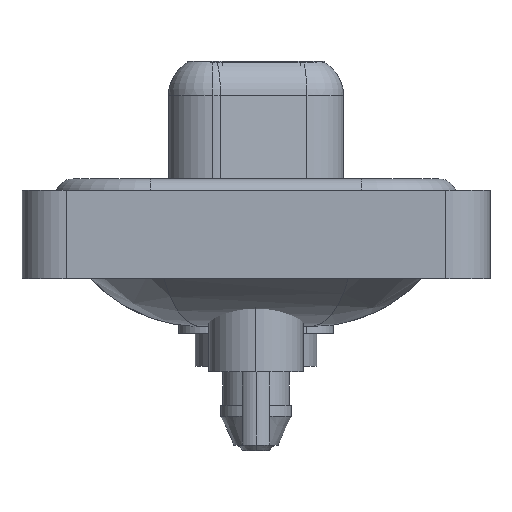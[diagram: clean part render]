
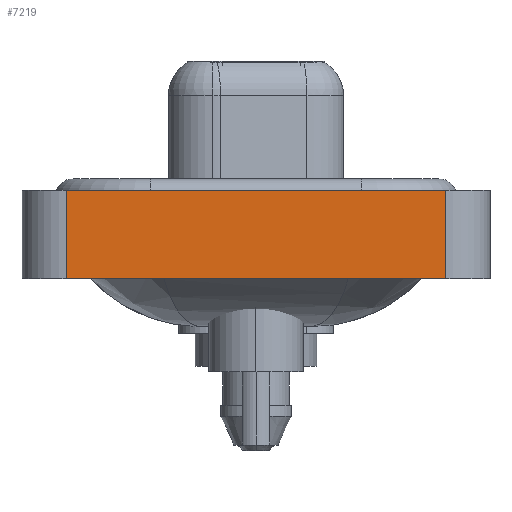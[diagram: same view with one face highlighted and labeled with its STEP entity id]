
A CAD part, left-side view. The second image highlights one B-rep face of the part: STEP entity #7219.
In plain terms, the highlighted planar face has unit normal (-1, 0, 0).
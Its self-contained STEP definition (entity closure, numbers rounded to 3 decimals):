
#433 = CARTESIAN_POINT ( 'NONE',  ( -7.25, 8.55, -3.6 ) ) ;
#957 = VERTEX_POINT ( 'NONE', #4955 ) ;
#996 = ORIENTED_EDGE ( 'NONE', *, *, #7742, .T. ) ;
#1111 = VERTEX_POINT ( 'NONE', #6572 ) ;
#1284 = FACE_OUTER_BOUND ( 'NONE', #15716, .T. ) ;
#1933 = VECTOR ( 'NONE', #14271, 1000. ) ;
#2251 = VERTEX_POINT ( 'NONE', #12895 ) ;
#2967 = CARTESIAN_POINT ( 'NONE',  ( -7.25, -8.55, -3.6 ) ) ;
#3525 = CARTESIAN_POINT ( 'NONE',  ( -7.25, -8.55, -3.6 ) ) ;
#4658 = CARTESIAN_POINT ( 'NONE',  ( -7.25, -8.55, 0.4 ) ) ;
#4955 = CARTESIAN_POINT ( 'NONE',  ( -7.25, -8.55, -3.6 ) ) ;
#5370 = ORIENTED_EDGE ( 'NONE', *, *, #6468, .F. ) ;
#6468 = EDGE_CURVE ( 'NONE', #1111, #2251, #15853, .T. ) ;
#6572 = CARTESIAN_POINT ( 'NONE',  ( -7.25, 8.55, 0.4 ) ) ;
#6816 = VECTOR ( 'NONE', #10041, 1000. ) ;
#7219 = ADVANCED_FACE ( 'NONE', ( #1284 ), #17560, .T. ) ;
#7633 = VECTOR ( 'NONE', #9516, 1000. ) ;
#7742 = EDGE_CURVE ( 'NONE', #9814, #957, #16306, .T. ) ;
#8198 = ORIENTED_EDGE ( 'NONE', *, *, #9485, .T. ) ;
#8516 = LINE ( 'NONE', #433, #10821 ) ;
#8829 = LINE ( 'NONE', #3525, #1933 ) ;
#9485 = EDGE_CURVE ( 'NONE', #957, #2251, #8829, .T. ) ;
#9516 = DIRECTION ( 'NONE',  ( 0., -1., 0. ) ) ;
#9814 = VERTEX_POINT ( 'NONE', #17172 ) ;
#10041 = DIRECTION ( 'NONE',  ( 0., -1., 0. ) ) ;
#10821 = VECTOR ( 'NONE', #16537, 1000. ) ;
#10858 = CARTESIAN_POINT ( 'NONE',  ( -7.25, -8.55, -3.6 ) ) ;
#10877 = DIRECTION ( 'NONE',  ( -1., 0., 0. ) ) ;
#12850 = EDGE_CURVE ( 'NONE', #9814, #1111, #8516, .T. ) ;
#12895 = CARTESIAN_POINT ( 'NONE',  ( -7.25, -8.55, 0.4 ) ) ;
#14271 = DIRECTION ( 'NONE',  ( 0., 0., 1. ) ) ;
#15403 = ORIENTED_EDGE ( 'NONE', *, *, #12850, .F. ) ;
#15716 = EDGE_LOOP ( 'NONE', ( #8198, #5370, #15403, #996 ) ) ;
#15853 = LINE ( 'NONE', #4658, #6816 ) ;
#16211 = AXIS2_PLACEMENT_3D ( 'NONE', #2967, #10877, #16409 ) ;
#16306 = LINE ( 'NONE', #10858, #7633 ) ;
#16409 = DIRECTION ( 'NONE',  ( 0., 0., 1. ) ) ;
#16537 = DIRECTION ( 'NONE',  ( 0., 0., 1. ) ) ;
#17172 = CARTESIAN_POINT ( 'NONE',  ( -7.25, 8.55, -3.6 ) ) ;
#17560 = PLANE ( 'NONE',  #16211 ) ;
